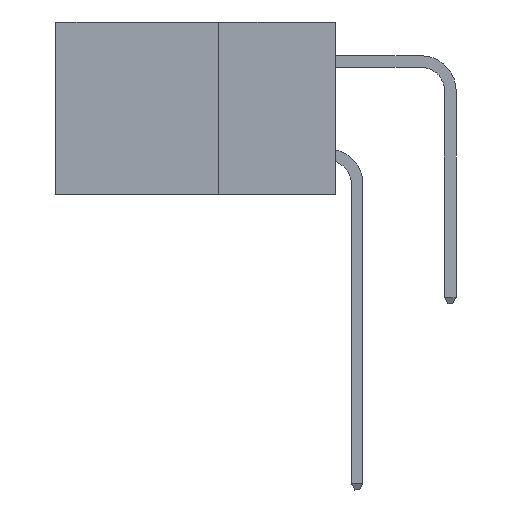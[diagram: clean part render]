
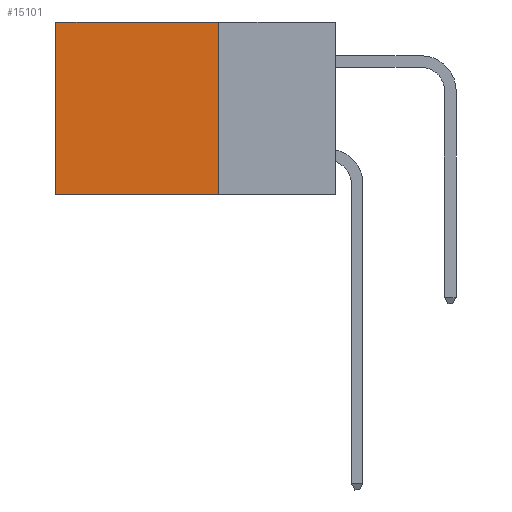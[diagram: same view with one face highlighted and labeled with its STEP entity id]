
A CAD part, left-side view. The second image highlights one B-rep face of the part: STEP entity #15101.
In plain terms, the highlighted planar face has unit normal (-1, 0, 0).
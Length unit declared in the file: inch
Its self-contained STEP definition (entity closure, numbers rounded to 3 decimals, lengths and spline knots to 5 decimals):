
#183 = ORIENTED_EDGE ( 'NONE', *, *, #15494, .F. ) ;
#311 = DIRECTION ( 'NONE',  ( 1., 0., 0. ) ) ;
#1009 = EDGE_LOOP ( 'NONE', ( #5025, #3374, #183, #13536 ) ) ;
#1773 = DIRECTION ( 'NONE',  ( 0., 0., -1. ) ) ;
#2861 = DIRECTION ( 'NONE',  ( 0., 1., 0. ) ) ;
#3374 = ORIENTED_EDGE ( 'NONE', *, *, #15437, .F. ) ;
#3734 = CARTESIAN_POINT ( 'NONE',  ( 0.2875, 0.25, 0. ) ) ;
#3822 = CARTESIAN_POINT ( 'NONE',  ( 0.2875, 0.6, 0. ) ) ;
#3961 = VERTEX_POINT ( 'NONE', #3822 ) ;
#4056 = DIRECTION ( 'NONE',  ( 0., 0., -1. ) ) ;
#4324 = VECTOR ( 'NONE', #2861, 39.37008 ) ;
#4635 = VECTOR ( 'NONE', #11056, 39.37008 ) ;
#5025 = ORIENTED_EDGE ( 'NONE', *, *, #13923, .T. ) ;
#5594 = VERTEX_POINT ( 'NONE', #3734 ) ;
#6910 = VECTOR ( 'NONE', #1773, 39.37008 ) ;
#7218 = LINE ( 'NONE', #11380, #4324 ) ;
#7325 = CARTESIAN_POINT ( 'NONE',  ( 0.2875, 0.6, -0.37 ) ) ;
#7526 = LINE ( 'NONE', #8335, #10852 ) ;
#8335 = CARTESIAN_POINT ( 'NONE',  ( 0.2875, 0.25, 0. ) ) ;
#8625 = CARTESIAN_POINT ( 'NONE',  ( 0.2875, 0.25, -0.37 ) ) ;
#8685 = VERTEX_POINT ( 'NONE', #8625 ) ;
#8904 = CARTESIAN_POINT ( 'NONE',  ( 0.2875, 0.25, 0. ) ) ;
#9634 = CARTESIAN_POINT ( 'NONE',  ( 0.2875, 0.25, -0.37 ) ) ;
#9973 = FACE_OUTER_BOUND ( 'NONE', #1009, .T. ) ;
#10350 = DIRECTION ( 'NONE',  ( 0., 0., -1. ) ) ;
#10852 = VECTOR ( 'NONE', #4056, 39.37008 ) ;
#11056 = DIRECTION ( 'NONE',  ( 0., 1., 0. ) ) ;
#11338 = AXIS2_PLACEMENT_3D ( 'NONE', #8904, #311, #10350 ) ;
#11380 = CARTESIAN_POINT ( 'NONE',  ( 0.2875, 0.25, 0. ) ) ;
#11760 = CARTESIAN_POINT ( 'NONE',  ( 0.2875, 0.6, 0. ) ) ;
#11875 = EDGE_CURVE ( 'NONE', #5594, #3961, #7218, .T. ) ;
#12621 = LINE ( 'NONE', #9634, #4635 ) ;
#13536 = ORIENTED_EDGE ( 'NONE', *, *, #11875, .T. ) ;
#13923 = EDGE_CURVE ( 'NONE', #3961, #14354, #14886, .T. ) ;
#14354 = VERTEX_POINT ( 'NONE', #7325 ) ;
#14886 = LINE ( 'NONE', #11760, #6910 ) ;
#15101 = ADVANCED_FACE ( 'NONE', ( #9973 ), #15853, .F. ) ;
#15437 = EDGE_CURVE ( 'NONE', #8685, #14354, #12621, .T. ) ;
#15494 = EDGE_CURVE ( 'NONE', #5594, #8685, #7526, .T. ) ;
#15853 = PLANE ( 'NONE',  #11338 ) ;
